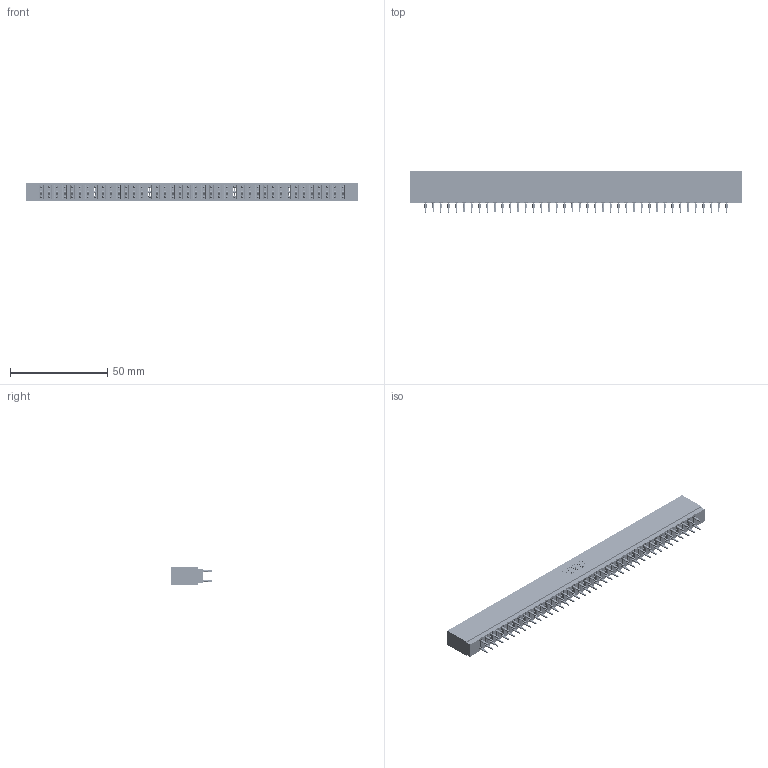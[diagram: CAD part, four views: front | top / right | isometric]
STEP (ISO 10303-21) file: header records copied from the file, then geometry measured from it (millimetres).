
FILE_DESCRIPTION (( 'STEP AP203' ), '1' );
FILE_NAME ('737-080-560-201.STEP', '2020-09-11T08:32:41', ( '' ), ( '' ), 'SwSTEP 2.0', 'SolidWorks 2020', '' );
FILE_SCHEMA (( 'CONFIG_CONTROL_DESIGN' ));
Length unit declared in the file: inch
Products named in the file (3): 737-080-560-201; 737 Part_Insulator Option - 01; 745-292-001_560
Assembly tree (81 placements, depth 2):
  737-080-560-201
    737 Part_Insulator Option - 01
    745-292-001_560  x80
Bounding box: 170.33 x 21.22 x 8.89 mm (x, y, z)
Volume: 17143.8 mm3; surface area: 26295.1 mm2
Topology: 81 solids, 81 shells, 8014 faces, 21935 edges, 13930 vertices
Faces by surface type: plane 4174, cylinder 1760, bspline 1600, torus 480
Entity records: 69230 total; most frequent: CARTESIAN_POINT 12523, ORIENTED_EDGE 11954, DIRECTION 10439, EDGE_CURVE 5977, VECTOR 5547, LINE 5547, VERTEX_POINT 3818, AXIS2_PLACEMENT_3D 2446
